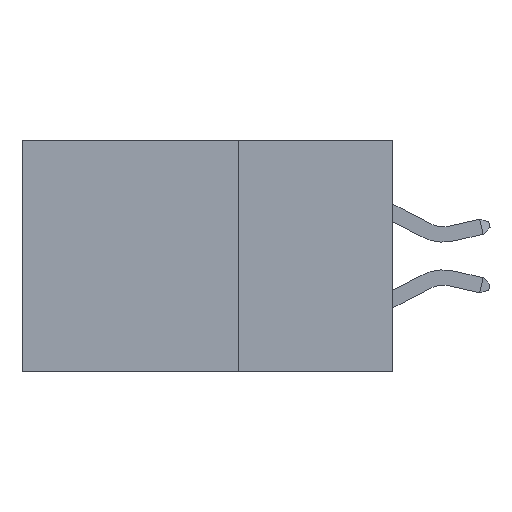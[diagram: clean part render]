
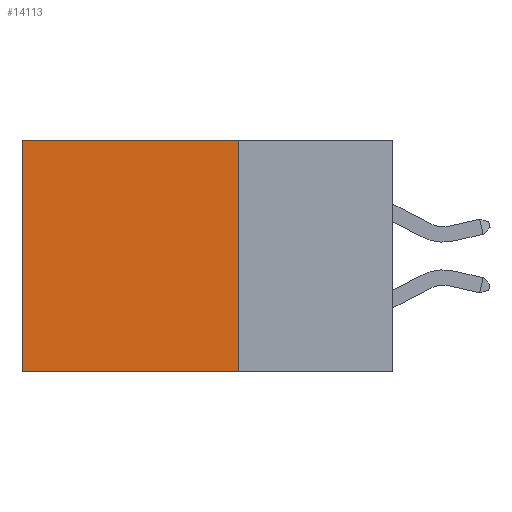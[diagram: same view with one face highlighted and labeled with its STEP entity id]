
A CAD part, left-side view. The second image highlights one B-rep face of the part: STEP entity #14113.
In plain terms, the highlighted planar face has unit normal (-1, 0, 0).
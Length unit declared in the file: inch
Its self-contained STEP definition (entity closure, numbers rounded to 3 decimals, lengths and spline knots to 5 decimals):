
#278 = LINE ( 'NONE', #13907, #10060 ) ;
#340 = AXIS2_PLACEMENT_3D ( 'NONE', #12217, #1628, #10916 ) ;
#618 = CARTESIAN_POINT ( 'NONE',  ( 0.2875, 0.6, -0.375 ) ) ;
#794 = VERTEX_POINT ( 'NONE', #11178 ) ;
#1543 = EDGE_LOOP ( 'NONE', ( #11064, #12380, #12749, #4513 ) ) ;
#1628 = DIRECTION ( 'NONE',  ( 1., 0., 0. ) ) ;
#2133 = LINE ( 'NONE', #618, #7548 ) ;
#2490 = VERTEX_POINT ( 'NONE', #6588 ) ;
#2861 = PLANE ( 'NONE',  #340 ) ;
#3063 = FACE_OUTER_BOUND ( 'NONE', #1543, .T. ) ;
#3373 = CARTESIAN_POINT ( 'NONE',  ( 0.2875, 0.25, -0.375 ) ) ;
#3607 = LINE ( 'NONE', #3373, #16218 ) ;
#4042 = CARTESIAN_POINT ( 'NONE',  ( 0.2875, 0.25, 0. ) ) ;
#4091 = CARTESIAN_POINT ( 'NONE',  ( 0.2875, 0.25, -0.375 ) ) ;
#4513 = ORIENTED_EDGE ( 'NONE', *, *, #6979, .T. ) ;
#5315 = DIRECTION ( 'NONE',  ( 0., 1., 0. ) ) ;
#6153 = DIRECTION ( 'NONE',  ( 0., 1., 0. ) ) ;
#6336 = CARTESIAN_POINT ( 'NONE',  ( 0.2875, 0.6, 0. ) ) ;
#6588 = CARTESIAN_POINT ( 'NONE',  ( 0.2875, 0.25, 0. ) ) ;
#6979 = EDGE_CURVE ( 'NONE', #2490, #9157, #12185, .T. ) ;
#7548 = VECTOR ( 'NONE', #12429, 39.37008 ) ;
#8335 = VERTEX_POINT ( 'NONE', #4091 ) ;
#9157 = VERTEX_POINT ( 'NONE', #6336 ) ;
#10060 = VECTOR ( 'NONE', #14016, 39.37008 ) ;
#10075 = EDGE_CURVE ( 'NONE', #8335, #794, #3607, .T. ) ;
#10387 = EDGE_CURVE ( 'NONE', #2490, #8335, #278, .T. ) ;
#10576 = VECTOR ( 'NONE', #5315, 39.37008 ) ;
#10916 = DIRECTION ( 'NONE',  ( 0., 0., -1. ) ) ;
#11064 = ORIENTED_EDGE ( 'NONE', *, *, #11282, .T. ) ;
#11178 = CARTESIAN_POINT ( 'NONE',  ( 0.2875, 0.6, -0.375 ) ) ;
#11282 = EDGE_CURVE ( 'NONE', #9157, #794, #2133, .T. ) ;
#12185 = LINE ( 'NONE', #4042, #10576 ) ;
#12217 = CARTESIAN_POINT ( 'NONE',  ( 0.2875, 0.25, -0.375 ) ) ;
#12380 = ORIENTED_EDGE ( 'NONE', *, *, #10075, .F. ) ;
#12429 = DIRECTION ( 'NONE',  ( 0., 0., -1. ) ) ;
#12749 = ORIENTED_EDGE ( 'NONE', *, *, #10387, .F. ) ;
#13907 = CARTESIAN_POINT ( 'NONE',  ( 0.2875, 0.25, -0.375 ) ) ;
#14016 = DIRECTION ( 'NONE',  ( 0., 0., -1. ) ) ;
#14113 = ADVANCED_FACE ( 'NONE', ( #3063 ), #2861, .F. ) ;
#16218 = VECTOR ( 'NONE', #6153, 39.37008 ) ;
